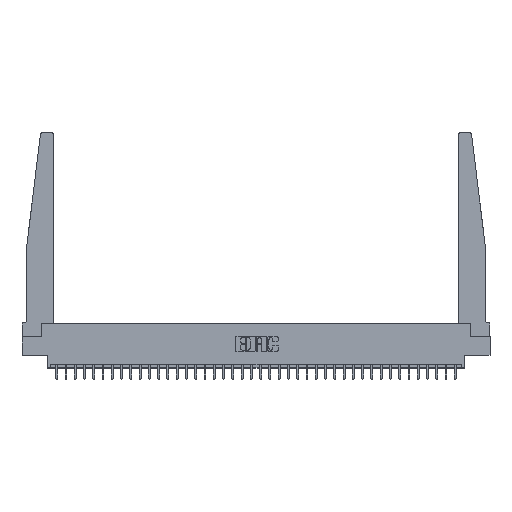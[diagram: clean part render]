
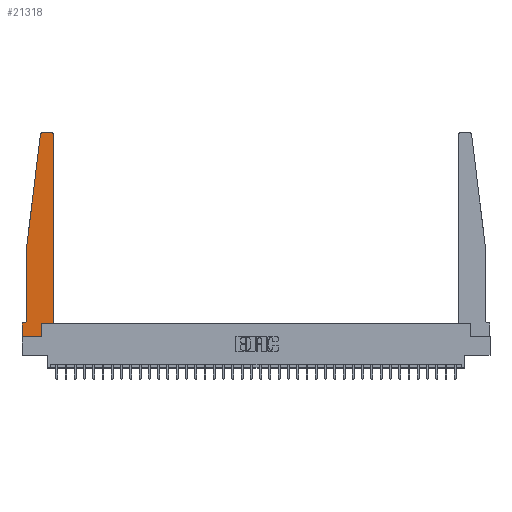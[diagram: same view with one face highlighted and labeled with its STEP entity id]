
A CAD part, top view. The second image highlights one B-rep face of the part: STEP entity #21318.
In plain terms, the highlighted planar face has unit normal (0, 0, 1).
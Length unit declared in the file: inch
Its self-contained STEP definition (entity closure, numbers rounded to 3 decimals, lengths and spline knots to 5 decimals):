
#148 = DIRECTION ( 'NONE',  ( 0., 0., -1. ) ) ;
#181 = LINE ( 'NONE', #20558, #10190 ) ;
#1232 = EDGE_LOOP ( 'NONE', ( #30058, #32707, #24269, #13930, #21022, #5332, #9238, #25519, #26189, #27542, #18373, #18068 ) ) ;
#1778 = CARTESIAN_POINT ( 'NONE',  ( 0., 0.1875, 0.37 ) ) ;
#1981 = VERTEX_POINT ( 'NONE', #2160 ) ;
#2160 = CARTESIAN_POINT ( 'NONE',  ( 0.015, 0.1875, 0.37 ) ) ;
#3099 = CARTESIAN_POINT ( 'NONE',  ( 0.395, 2.75, 0.37 ) ) ;
#3254 = LINE ( 'NONE', #21582, #33525 ) ;
#3716 = CIRCLE ( 'NONE', #22875, 0.03 ) ;
#4642 = FACE_OUTER_BOUND ( 'NONE', #1232, .T. ) ;
#5206 = AXIS2_PLACEMENT_3D ( 'NONE', #23597, #148, #31982 ) ;
#5332 = ORIENTED_EDGE ( 'NONE', *, *, #27549, .T. ) ;
#5780 = CIRCLE ( 'NONE', #5206, 0.05 ) ;
#5790 = CARTESIAN_POINT ( 'NONE',  ( 0.065, 0.2375, 0.37 ) ) ;
#7114 = VERTEX_POINT ( 'NONE', #31353 ) ;
#7131 = EDGE_CURVE ( 'NONE', #8545, #21465, #181, .T. ) ;
#7186 = VERTEX_POINT ( 'NONE', #13211 ) ;
#7274 = CARTESIAN_POINT ( 'NONE',  ( 0.065, 0.1875, 0.37 ) ) ;
#8413 = CARTESIAN_POINT ( 'NONE',  ( 0.2605, 0., 0.37 ) ) ;
#8545 = VERTEX_POINT ( 'NONE', #8413 ) ;
#9238 = ORIENTED_EDGE ( 'NONE', *, *, #13355, .T. ) ;
#9704 = VECTOR ( 'NONE', #16359, 39.37008 ) ;
#9833 = DIRECTION ( 'NONE',  ( -1., 0., 0. ) ) ;
#10098 = VERTEX_POINT ( 'NONE', #29256 ) ;
#10134 = CARTESIAN_POINT ( 'NONE',  ( 0.425, 0.18, 0.37 ) ) ;
#10190 = VECTOR ( 'NONE', #26045, 39.37008 ) ;
#10277 = LINE ( 'NONE', #20686, #11260 ) ;
#10661 = DIRECTION ( 'NONE',  ( 0., 0., 1. ) ) ;
#11260 = VECTOR ( 'NONE', #31143, 39.37008 ) ;
#11325 = VECTOR ( 'NONE', #9833, 39.37008 ) ;
#11642 = CARTESIAN_POINT ( 'NONE',  ( 0.24675, 2.72367, 0.37 ) ) ;
#13050 = PLANE ( 'NONE',  #14655 ) ;
#13172 = DIRECTION ( 'NONE',  ( 0., 1., 0. ) ) ;
#13211 = CARTESIAN_POINT ( 'NONE',  ( 0.425, 0.18, 0.37 ) ) ;
#13355 = EDGE_CURVE ( 'NONE', #28036, #7114, #3254, .T. ) ;
#13602 = CARTESIAN_POINT ( 'NONE',  ( 0.065, 1.25, 0.37 ) ) ;
#13930 = ORIENTED_EDGE ( 'NONE', *, *, #17010, .T. ) ;
#14295 = CARTESIAN_POINT ( 'NONE',  ( 0., 0., 0.37 ) ) ;
#14655 = AXIS2_PLACEMENT_3D ( 'NONE', #26052, #10661, #23301 ) ;
#15056 = VECTOR ( 'NONE', #22684, 39.37008 ) ;
#15159 = VECTOR ( 'NONE', #17301, 39.37008 ) ;
#15714 = VECTOR ( 'NONE', #24782, 39.37008 ) ;
#16359 = DIRECTION ( 'NONE',  ( 1., 0., 0. ) ) ;
#16449 = CARTESIAN_POINT ( 'NONE',  ( 0.2605, 0.18, 0.37 ) ) ;
#17010 = EDGE_CURVE ( 'NONE', #27798, #17037, #10277, .T. ) ;
#17037 = VERTEX_POINT ( 'NONE', #5790 ) ;
#17050 = DIRECTION ( 'NONE',  ( 1., 0., 0. ) ) ;
#17301 = DIRECTION ( 'NONE',  ( 1., 0., 0. ) ) ;
#18068 = ORIENTED_EDGE ( 'NONE', *, *, #27521, .T. ) ;
#18085 = VERTEX_POINT ( 'NONE', #27096 ) ;
#18373 = ORIENTED_EDGE ( 'NONE', *, *, #20029, .T. ) ;
#18378 = EDGE_CURVE ( 'NONE', #17037, #1981, #5780, .T. ) ;
#19638 = DIRECTION ( 'NONE',  ( 0., 0., 1. ) ) ;
#20029 = EDGE_CURVE ( 'NONE', #7186, #10098, #31315, .T. ) ;
#20293 = LINE ( 'NONE', #7274, #15056 ) ;
#20558 = CARTESIAN_POINT ( 'NONE',  ( 0.2605, 0.18, 0.37 ) ) ;
#20561 = EDGE_CURVE ( 'NONE', #7114, #8545, #29205, .T. ) ;
#20686 = CARTESIAN_POINT ( 'NONE',  ( 0.065, 1.25, 0.37 ) ) ;
#21022 = ORIENTED_EDGE ( 'NONE', *, *, #18378, .T. ) ;
#21318 = ADVANCED_FACE ( 'NONE', ( #4642 ), #13050, .T. ) ;
#21465 = VERTEX_POINT ( 'NONE', #16449 ) ;
#21582 = CARTESIAN_POINT ( 'NONE',  ( 0., 0., 0.37 ) ) ;
#22140 = AXIS2_PLACEMENT_3D ( 'NONE', #32612, #19638, #17050 ) ;
#22684 = DIRECTION ( 'NONE',  ( -1., 0., 0. ) ) ;
#22875 = AXIS2_PLACEMENT_3D ( 'NONE', #30093, #32462, #27171 ) ;
#23301 = DIRECTION ( 'NONE',  ( 1., 0., 0. ) ) ;
#23597 = CARTESIAN_POINT ( 'NONE',  ( 0.015, 0.2375, 0.37 ) ) ;
#24269 = ORIENTED_EDGE ( 'NONE', *, *, #32058, .T. ) ;
#24397 = VECTOR ( 'NONE', #13172, 39.37008 ) ;
#24437 = LINE ( 'NONE', #27538, #15714 ) ;
#24782 = DIRECTION ( 'NONE',  ( -0.122, -0.992, 0. ) ) ;
#25519 = ORIENTED_EDGE ( 'NONE', *, *, #20561, .T. ) ;
#26045 = DIRECTION ( 'NONE',  ( 0., 1., 0. ) ) ;
#26052 = CARTESIAN_POINT ( 'NONE',  ( 0., 0.1875, 0.37 ) ) ;
#26189 = ORIENTED_EDGE ( 'NONE', *, *, #7131, .T. ) ;
#26334 = CARTESIAN_POINT ( 'NONE',  ( 0.425, 0.18, 0.37 ) ) ;
#27096 = CARTESIAN_POINT ( 'NONE',  ( 0.27653, 2.75, 0.37 ) ) ;
#27171 = DIRECTION ( 'NONE',  ( 1., 0., 0. ) ) ;
#27521 = EDGE_CURVE ( 'NONE', #10098, #30950, #33630, .T. ) ;
#27538 = CARTESIAN_POINT ( 'NONE',  ( 0.065, 1.25, 0.37 ) ) ;
#27542 = ORIENTED_EDGE ( 'NONE', *, *, #29807, .T. ) ;
#27549 = EDGE_CURVE ( 'NONE', #1981, #28036, #20293, .T. ) ;
#27798 = VERTEX_POINT ( 'NONE', #13602 ) ;
#28036 = VERTEX_POINT ( 'NONE', #1778 ) ;
#28083 = LINE ( 'NONE', #10134, #15159 ) ;
#29205 = LINE ( 'NONE', #14295, #9704 ) ;
#29256 = CARTESIAN_POINT ( 'NONE',  ( 0.425, 2.72, 0.37 ) ) ;
#29305 = DIRECTION ( 'NONE',  ( 0., -1., 0. ) ) ;
#29446 = EDGE_CURVE ( 'NONE', #30950, #18085, #33263, .T. ) ;
#29807 = EDGE_CURVE ( 'NONE', #21465, #7186, #28083, .T. ) ;
#30058 = ORIENTED_EDGE ( 'NONE', *, *, #29446, .T. ) ;
#30093 = CARTESIAN_POINT ( 'NONE',  ( 0.27653, 2.72, 0.37 ) ) ;
#30201 = VERTEX_POINT ( 'NONE', #11642 ) ;
#30950 = VERTEX_POINT ( 'NONE', #3099 ) ;
#31040 = CARTESIAN_POINT ( 'NONE',  ( 0.25, 2.75, 0.37 ) ) ;
#31143 = DIRECTION ( 'NONE',  ( 0., -1., 0. ) ) ;
#31315 = LINE ( 'NONE', #26334, #24397 ) ;
#31353 = CARTESIAN_POINT ( 'NONE',  ( 0., 0., 0.37 ) ) ;
#31982 = DIRECTION ( 'NONE',  ( -1., 0., 0. ) ) ;
#32058 = EDGE_CURVE ( 'NONE', #30201, #27798, #24437, .T. ) ;
#32462 = DIRECTION ( 'NONE',  ( 0., 0., 1. ) ) ;
#32612 = CARTESIAN_POINT ( 'NONE',  ( 0.395, 2.72, 0.37 ) ) ;
#32707 = ORIENTED_EDGE ( 'NONE', *, *, #33724, .T. ) ;
#33263 = LINE ( 'NONE', #31040, #11325 ) ;
#33525 = VECTOR ( 'NONE', #29305, 39.37008 ) ;
#33630 = CIRCLE ( 'NONE', #22140, 0.03 ) ;
#33724 = EDGE_CURVE ( 'NONE', #18085, #30201, #3716, .T. ) ;
